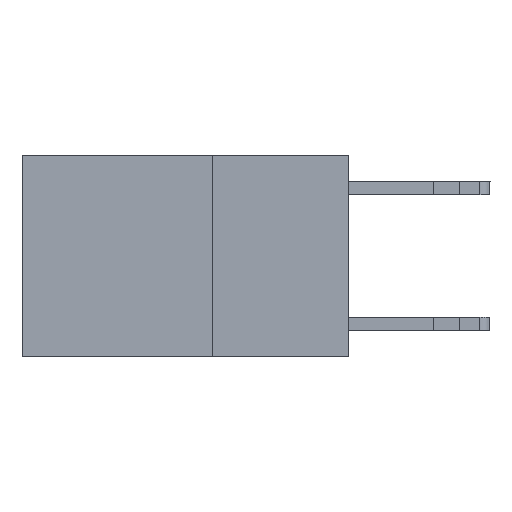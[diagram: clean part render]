
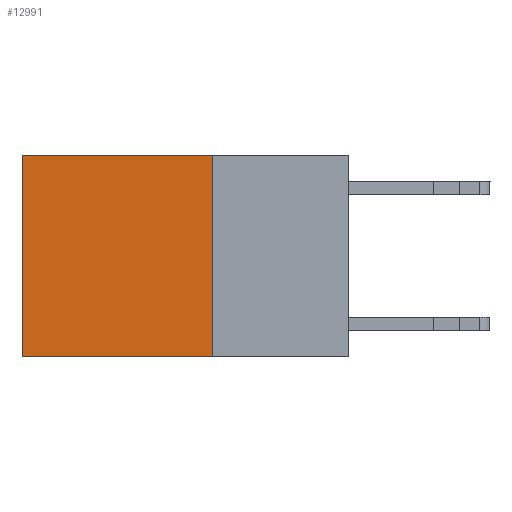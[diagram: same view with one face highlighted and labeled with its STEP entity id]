
A CAD part, left-side view. The second image highlights one B-rep face of the part: STEP entity #12991.
In plain terms, the highlighted planar face has unit normal (-1, 0, 0).
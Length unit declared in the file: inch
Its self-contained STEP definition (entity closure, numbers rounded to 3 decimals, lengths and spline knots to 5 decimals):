
#440 = LINE ( 'NONE', #4937, #5066 ) ;
#796 = CARTESIAN_POINT ( 'NONE',  ( 0.2625, 0.25, -0.37 ) ) ;
#1250 = EDGE_CURVE ( 'NONE', #5037, #5135, #4759, .T. ) ;
#1280 = CARTESIAN_POINT ( 'NONE',  ( 0.2625, 0.25, 0. ) ) ;
#1534 = EDGE_LOOP ( 'NONE', ( #14277, #13673, #8174, #13463 ) ) ;
#1624 = EDGE_CURVE ( 'NONE', #5037, #11461, #8144, .T. ) ;
#2646 = LINE ( 'NONE', #7067, #8923 ) ;
#3573 = EDGE_CURVE ( 'NONE', #11461, #4780, #440, .T. ) ;
#4141 = PLANE ( 'NONE',  #6626 ) ;
#4293 = DIRECTION ( 'NONE',  ( 1., 0., 0. ) ) ;
#4759 = LINE ( 'NONE', #8237, #11184 ) ;
#4780 = VERTEX_POINT ( 'NONE', #11629 ) ;
#4937 = CARTESIAN_POINT ( 'NONE',  ( 0.2625, 0.25, -0.37 ) ) ;
#5037 = VERTEX_POINT ( 'NONE', #6330 ) ;
#5066 = VECTOR ( 'NONE', #9444, 39.37008 ) ;
#5135 = VERTEX_POINT ( 'NONE', #5729 ) ;
#5729 = CARTESIAN_POINT ( 'NONE',  ( 0.2625, 0.6, 0. ) ) ;
#6094 = DIRECTION ( 'NONE',  ( 0., 0., -1. ) ) ;
#6330 = CARTESIAN_POINT ( 'NONE',  ( 0.2625, 0.25, 0. ) ) ;
#6462 = VECTOR ( 'NONE', #9025, 39.37008 ) ;
#6626 = AXIS2_PLACEMENT_3D ( 'NONE', #10024, #4293, #13415 ) ;
#7067 = CARTESIAN_POINT ( 'NONE',  ( 0.2625, 0.6, 0. ) ) ;
#8144 = LINE ( 'NONE', #1280, #6462 ) ;
#8174 = ORIENTED_EDGE ( 'NONE', *, *, #1624, .F. ) ;
#8237 = CARTESIAN_POINT ( 'NONE',  ( 0.2625, 0.25, 0. ) ) ;
#8516 = EDGE_CURVE ( 'NONE', #5135, #4780, #2646, .T. ) ;
#8923 = VECTOR ( 'NONE', #6094, 39.37008 ) ;
#9025 = DIRECTION ( 'NONE',  ( 0., 0., -1. ) ) ;
#9444 = DIRECTION ( 'NONE',  ( 0., 1., 0. ) ) ;
#9727 = FACE_OUTER_BOUND ( 'NONE', #1534, .T. ) ;
#10024 = CARTESIAN_POINT ( 'NONE',  ( 0.2625, 0.25, 0. ) ) ;
#11184 = VECTOR ( 'NONE', #11320, 39.37008 ) ;
#11320 = DIRECTION ( 'NONE',  ( 0., 1., 0. ) ) ;
#11461 = VERTEX_POINT ( 'NONE', #796 ) ;
#11629 = CARTESIAN_POINT ( 'NONE',  ( 0.2625, 0.6, -0.37 ) ) ;
#12991 = ADVANCED_FACE ( 'NONE', ( #9727 ), #4141, .F. ) ;
#13415 = DIRECTION ( 'NONE',  ( 0., 0., -1. ) ) ;
#13463 = ORIENTED_EDGE ( 'NONE', *, *, #1250, .T. ) ;
#13673 = ORIENTED_EDGE ( 'NONE', *, *, #3573, .F. ) ;
#14277 = ORIENTED_EDGE ( 'NONE', *, *, #8516, .T. ) ;
